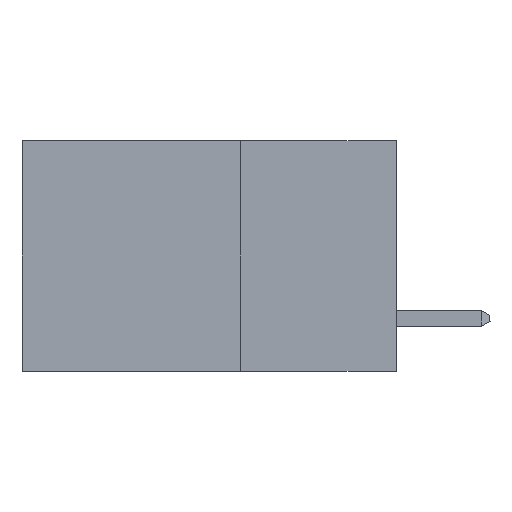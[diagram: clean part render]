
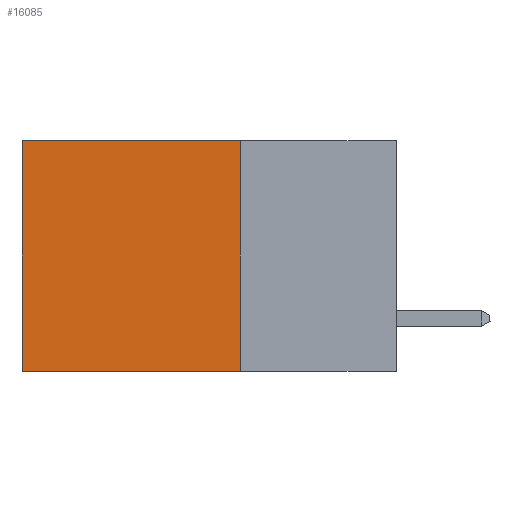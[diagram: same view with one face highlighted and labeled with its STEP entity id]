
A CAD part, left-side view. The second image highlights one B-rep face of the part: STEP entity #16085.
In plain terms, the highlighted planar face has unit normal (-1, 0, 0).
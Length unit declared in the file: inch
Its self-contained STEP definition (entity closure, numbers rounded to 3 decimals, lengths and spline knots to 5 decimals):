
#151 = LINE ( 'NONE', #14172, #4919 ) ;
#680 = VECTOR ( 'NONE', #6640, 39.37008 ) ;
#835 = EDGE_CURVE ( 'NONE', #12577, #15312, #3948, .T. ) ;
#1064 = ORIENTED_EDGE ( 'NONE', *, *, #6499, .F. ) ;
#1237 = EDGE_CURVE ( 'NONE', #18326, #15312, #151, .T. ) ;
#2348 = CARTESIAN_POINT ( 'NONE',  ( 0.298, 0.25, 0. ) ) ;
#2652 = AXIS2_PLACEMENT_3D ( 'NONE', #2348, #16888, #11942 ) ;
#2933 = CARTESIAN_POINT ( 'NONE',  ( 0.298, 0.6, 0. ) ) ;
#3948 = LINE ( 'NONE', #14747, #6708 ) ;
#4785 = LINE ( 'NONE', #19389, #6559 ) ;
#4919 = VECTOR ( 'NONE', #15761, 39.37008 ) ;
#5158 = FACE_OUTER_BOUND ( 'NONE', #16259, .T. ) ;
#6442 = LINE ( 'NONE', #19315, #680 ) ;
#6499 = EDGE_CURVE ( 'NONE', #11466, #18326, #4785, .T. ) ;
#6559 = VECTOR ( 'NONE', #11194, 39.37008 ) ;
#6640 = DIRECTION ( 'NONE',  ( 0., 1., 0. ) ) ;
#6708 = VECTOR ( 'NONE', #12919, 39.37008 ) ;
#6857 = CARTESIAN_POINT ( 'NONE',  ( 0.298, 0.6, -0.37 ) ) ;
#8202 = ORIENTED_EDGE ( 'NONE', *, *, #835, .T. ) ;
#8311 = ORIENTED_EDGE ( 'NONE', *, *, #9626, .T. ) ;
#9626 = EDGE_CURVE ( 'NONE', #11466, #12577, #6442, .T. ) ;
#11194 = DIRECTION ( 'NONE',  ( 0., 0., -1. ) ) ;
#11466 = VERTEX_POINT ( 'NONE', #12879 ) ;
#11942 = DIRECTION ( 'NONE',  ( 0., 0., -1. ) ) ;
#12577 = VERTEX_POINT ( 'NONE', #2933 ) ;
#12879 = CARTESIAN_POINT ( 'NONE',  ( 0.298, 0.25, 0. ) ) ;
#12919 = DIRECTION ( 'NONE',  ( 0., 0., -1. ) ) ;
#13355 = ORIENTED_EDGE ( 'NONE', *, *, #1237, .F. ) ;
#14172 = CARTESIAN_POINT ( 'NONE',  ( 0.298, 0.25, -0.37 ) ) ;
#14747 = CARTESIAN_POINT ( 'NONE',  ( 0.298, 0.6, 0. ) ) ;
#15312 = VERTEX_POINT ( 'NONE', #6857 ) ;
#15761 = DIRECTION ( 'NONE',  ( 0., 1., 0. ) ) ;
#16037 = CARTESIAN_POINT ( 'NONE',  ( 0.298, 0.25, -0.37 ) ) ;
#16085 = ADVANCED_FACE ( 'NONE', ( #5158 ), #18248, .F. ) ;
#16259 = EDGE_LOOP ( 'NONE', ( #8202, #13355, #1064, #8311 ) ) ;
#16888 = DIRECTION ( 'NONE',  ( 1., 0., 0. ) ) ;
#18248 = PLANE ( 'NONE',  #2652 ) ;
#18326 = VERTEX_POINT ( 'NONE', #16037 ) ;
#19315 = CARTESIAN_POINT ( 'NONE',  ( 0.298, 0.25, 0. ) ) ;
#19389 = CARTESIAN_POINT ( 'NONE',  ( 0.298, 0.25, 0. ) ) ;
